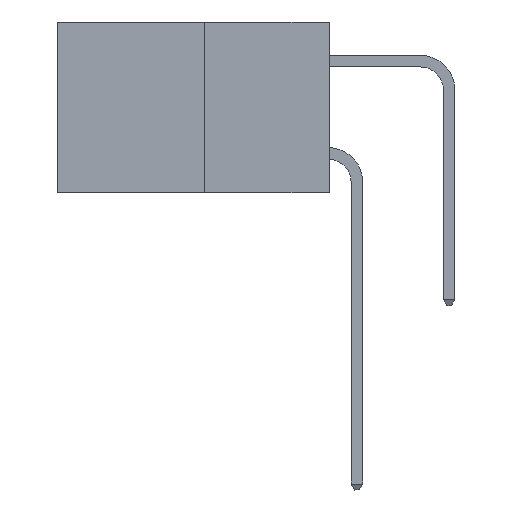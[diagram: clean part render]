
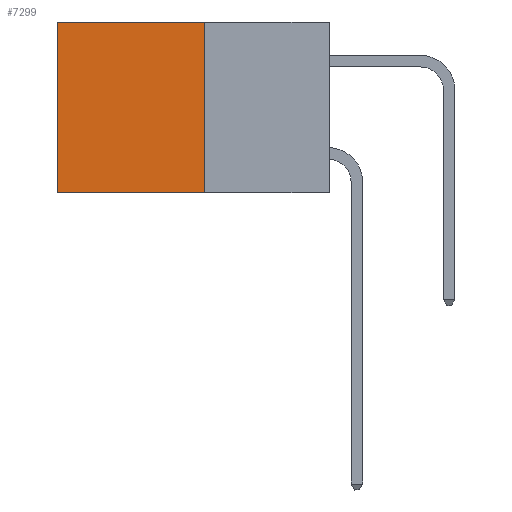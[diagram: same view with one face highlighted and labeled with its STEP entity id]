
A CAD part, left-side view. The second image highlights one B-rep face of the part: STEP entity #7299.
In plain terms, the highlighted planar face has unit normal (-1, 0, 0).
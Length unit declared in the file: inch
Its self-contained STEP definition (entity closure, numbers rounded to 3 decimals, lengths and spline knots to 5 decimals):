
#19 = CARTESIAN_POINT ( 'NONE',  ( 0.277, 0.27, -0.37 ) ) ;
#480 = FACE_OUTER_BOUND ( 'NONE', #18803, .T. ) ;
#491 = DIRECTION ( 'NONE',  ( 0., 0., -1. ) ) ;
#758 = DIRECTION ( 'NONE',  ( 0., 1., 0. ) ) ;
#1324 = DIRECTION ( 'NONE',  ( 0., 0., -1. ) ) ;
#2557 = CARTESIAN_POINT ( 'NONE',  ( 0.277, 0.27, 0. ) ) ;
#3155 = DIRECTION ( 'NONE',  ( 0., 0., -1. ) ) ;
#3180 = DIRECTION ( 'NONE',  ( 1., 0., 0. ) ) ;
#3271 = PLANE ( 'NONE',  #13265 ) ;
#3432 = CARTESIAN_POINT ( 'NONE',  ( 0.277, 0.27, -0.37 ) ) ;
#3783 = ORIENTED_EDGE ( 'NONE', *, *, #17782, .F. ) ;
#4800 = EDGE_CURVE ( 'NONE', #13575, #22680, #20889, .T. ) ;
#5151 = CARTESIAN_POINT ( 'NONE',  ( 0.277, 0.59, -0.37 ) ) ;
#6471 = VERTEX_POINT ( 'NONE', #24054 ) ;
#7271 = LINE ( 'NONE', #23203, #16688 ) ;
#7286 = CARTESIAN_POINT ( 'NONE',  ( 0.277, 0.59, -0.37 ) ) ;
#7299 = ADVANCED_FACE ( 'NONE', ( #480 ), #3271, .F. ) ;
#8098 = LINE ( 'NONE', #21919, #20660 ) ;
#8904 = DIRECTION ( 'NONE',  ( 0., 1., 0. ) ) ;
#10688 = EDGE_CURVE ( 'NONE', #13575, #6471, #8098, .T. ) ;
#11012 = VECTOR ( 'NONE', #491, 39.37008 ) ;
#13265 = AXIS2_PLACEMENT_3D ( 'NONE', #3432, #3180, #3155 ) ;
#13575 = VERTEX_POINT ( 'NONE', #2557 ) ;
#14894 = VECTOR ( 'NONE', #1324, 39.37008 ) ;
#15485 = LINE ( 'NONE', #5151, #14894 ) ;
#16688 = VECTOR ( 'NONE', #758, 39.37008 ) ;
#17350 = VERTEX_POINT ( 'NONE', #7286 ) ;
#17782 = EDGE_CURVE ( 'NONE', #22680, #17350, #7271, .T. ) ;
#18544 = ORIENTED_EDGE ( 'NONE', *, *, #10688, .T. ) ;
#18803 = EDGE_LOOP ( 'NONE', ( #20246, #3783, #19091, #18544 ) ) ;
#19091 = ORIENTED_EDGE ( 'NONE', *, *, #4800, .F. ) ;
#20246 = ORIENTED_EDGE ( 'NONE', *, *, #22016, .T. ) ;
#20660 = VECTOR ( 'NONE', #8904, 39.37008 ) ;
#20889 = LINE ( 'NONE', #19, #11012 ) ;
#21825 = CARTESIAN_POINT ( 'NONE',  ( 0.277, 0.27, -0.37 ) ) ;
#21919 = CARTESIAN_POINT ( 'NONE',  ( 0.277, 0.27, 0. ) ) ;
#22016 = EDGE_CURVE ( 'NONE', #6471, #17350, #15485, .T. ) ;
#22680 = VERTEX_POINT ( 'NONE', #21825 ) ;
#23203 = CARTESIAN_POINT ( 'NONE',  ( 0.277, 0.27, -0.37 ) ) ;
#24054 = CARTESIAN_POINT ( 'NONE',  ( 0.277, 0.59, 0. ) ) ;
